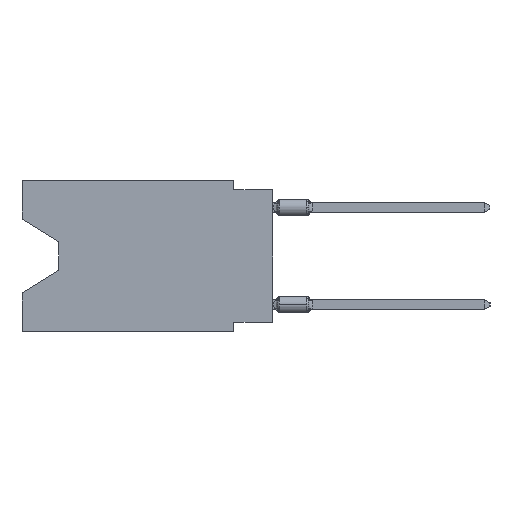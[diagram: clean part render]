
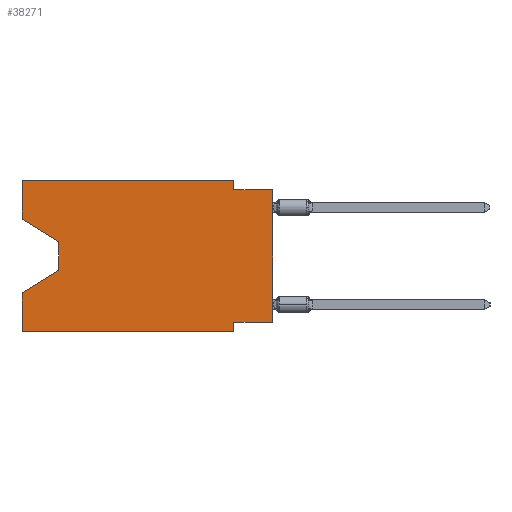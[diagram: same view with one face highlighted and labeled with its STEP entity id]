
A CAD part, left-side view. The second image highlights one B-rep face of the part: STEP entity #38271.
In plain terms, the highlighted planar face has unit normal (-1, 0, 0).
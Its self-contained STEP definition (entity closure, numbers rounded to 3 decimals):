
#84 = AXIS2_PLACEMENT_3D ( 'NONE', #37325, #18719, #42147 ) ;
#248 = EDGE_CURVE ( 'NONE', #34217, #11226, #20038, .T. ) ;
#250 = LINE ( 'NONE', #18867, #55713 ) ;
#2290 = VECTOR ( 'NONE', #35414, 1000. ) ;
#2906 = EDGE_CURVE ( 'NONE', #6430, #59969, #56478, .T. ) ;
#4871 = ORIENTED_EDGE ( 'NONE', *, *, #248, .T. ) ;
#5699 = CARTESIAN_POINT ( 'NONE',  ( 0., 0., 0. ) ) ;
#5927 = CARTESIAN_POINT ( 'NONE',  ( 0., 13.97, -4.013 ) ) ;
#6006 = LINE ( 'NONE', #5699, #39794 ) ;
#6430 = VERTEX_POINT ( 'NONE', #25200 ) ;
#6886 = EDGE_CURVE ( 'NONE', #49086, #6430, #51984, .T. ) ;
#7546 = EDGE_CURVE ( 'NONE', #26648, #34217, #13705, .T. ) ;
#8816 = DIRECTION ( 'NONE',  ( 0., 0.855, -0.519 ) ) ;
#9504 = VERTEX_POINT ( 'NONE', #32286 ) ;
#11226 = VERTEX_POINT ( 'NONE', #53431 ) ;
#12006 = DIRECTION ( 'NONE',  ( 0., 0., -1. ) ) ;
#13421 = CARTESIAN_POINT ( 'NONE',  ( 0., 2.54, -9.271 ) ) ;
#13705 = LINE ( 'NONE', #24275, #27779 ) ;
#13907 = FACE_OUTER_BOUND ( 'NONE', #61934, .T. ) ;
#14045 = CARTESIAN_POINT ( 'NONE',  ( 0., 16.383, -9.906 ) ) ;
#15239 = VECTOR ( 'NONE', #28794, 1000. ) ;
#15322 = DIRECTION ( 'NONE',  ( 0., 0., -1. ) ) ;
#15374 = VECTOR ( 'NONE', #35483, 1000. ) ;
#16225 = CARTESIAN_POINT ( 'NONE',  ( 0., 16.383, -2.546 ) ) ;
#17787 = ORIENTED_EDGE ( 'NONE', *, *, #36346, .T. ) ;
#17876 = ORIENTED_EDGE ( 'NONE', *, *, #55189, .F. ) ;
#18494 = ORIENTED_EDGE ( 'NONE', *, *, #45465, .T. ) ;
#18719 = DIRECTION ( 'NONE',  ( 1., 0., 0. ) ) ;
#18867 = CARTESIAN_POINT ( 'NONE',  ( 0., 2.54, -9.906 ) ) ;
#19535 = VERTEX_POINT ( 'NONE', #13421 ) ;
#20038 = LINE ( 'NONE', #63069, #56953 ) ;
#20681 = CARTESIAN_POINT ( 'NONE',  ( 0., 16.383, -9.906 ) ) ;
#22104 = EDGE_CURVE ( 'NONE', #9504, #36078, #6006, .T. ) ;
#22663 = ORIENTED_EDGE ( 'NONE', *, *, #22104, .T. ) ;
#22854 = CARTESIAN_POINT ( 'NONE',  ( 0., 2.54, -9.906 ) ) ;
#24275 = CARTESIAN_POINT ( 'NONE',  ( 0., 13.97, -4.013 ) ) ;
#24982 = VECTOR ( 'NONE', #48238, 1000. ) ;
#25200 = CARTESIAN_POINT ( 'NONE',  ( 0., 16.383, 0. ) ) ;
#26648 = VERTEX_POINT ( 'NONE', #5927 ) ;
#27779 = VECTOR ( 'NONE', #32630, 1000. ) ;
#28009 = EDGE_CURVE ( 'NONE', #19535, #44977, #250, .T. ) ;
#28794 = DIRECTION ( 'NONE',  ( 0., -1., 0. ) ) ;
#28834 = ORIENTED_EDGE ( 'NONE', *, *, #48474, .F. ) ;
#29597 = CARTESIAN_POINT ( 'NONE',  ( 0., 0., -0.635 ) ) ;
#30302 = CARTESIAN_POINT ( 'NONE',  ( 0., 16.383, 0. ) ) ;
#30647 = LINE ( 'NONE', #60180, #42364 ) ;
#32067 = DIRECTION ( 'NONE',  ( 0., -1., 0. ) ) ;
#32108 = LINE ( 'NONE', #30302, #2290 ) ;
#32286 = CARTESIAN_POINT ( 'NONE',  ( 0., 0., -9.271 ) ) ;
#32630 = DIRECTION ( 'NONE',  ( 0., 0., -1. ) ) ;
#33446 = CARTESIAN_POINT ( 'NONE',  ( 0., 13.97, -5.893 ) ) ;
#33474 = PLANE ( 'NONE',  #84 ) ;
#33512 = CARTESIAN_POINT ( 'NONE',  ( 0., 2.54, 0. ) ) ;
#34217 = VERTEX_POINT ( 'NONE', #33446 ) ;
#35414 = DIRECTION ( 'NONE',  ( 0., 0., 1. ) ) ;
#35483 = DIRECTION ( 'NONE',  ( 0., -0.855, -0.519 ) ) ;
#35676 = VECTOR ( 'NONE', #32067, 1000. ) ;
#36078 = VERTEX_POINT ( 'NONE', #54875 ) ;
#36346 = EDGE_CURVE ( 'NONE', #36873, #44977, #58024, .T. ) ;
#36873 = VERTEX_POINT ( 'NONE', #20681 ) ;
#37325 = CARTESIAN_POINT ( 'NONE',  ( 0., 16.383, 0. ) ) ;
#38271 = ADVANCED_FACE ( 'NONE', ( #13907 ), #33474, .F. ) ;
#39794 = VECTOR ( 'NONE', #44228, 1000. ) ;
#41596 = VECTOR ( 'NONE', #60967, 1000. ) ;
#42023 = DIRECTION ( 'NONE',  ( 0., 0., 1. ) ) ;
#42147 = DIRECTION ( 'NONE',  ( 0., 0., -1. ) ) ;
#42364 = VECTOR ( 'NONE', #12006, 1000. ) ;
#43428 = LINE ( 'NONE', #29597, #24982 ) ;
#44228 = DIRECTION ( 'NONE',  ( 0., 0., 1. ) ) ;
#44977 = VERTEX_POINT ( 'NONE', #22854 ) ;
#45465 = EDGE_CURVE ( 'NONE', #49086, #26648, #55715, .T. ) ;
#46901 = ORIENTED_EDGE ( 'NONE', *, *, #50040, .F. ) ;
#48196 = ORIENTED_EDGE ( 'NONE', *, *, #7546, .T. ) ;
#48238 = DIRECTION ( 'NONE',  ( 0., -1., 0. ) ) ;
#48474 = EDGE_CURVE ( 'NONE', #36873, #11226, #32108, .T. ) ;
#49086 = VERTEX_POINT ( 'NONE', #61565 ) ;
#50040 = EDGE_CURVE ( 'NONE', #50579, #36078, #43428, .T. ) ;
#50389 = LINE ( 'NONE', #50703, #41596 ) ;
#50579 = VERTEX_POINT ( 'NONE', #56041 ) ;
#50703 = CARTESIAN_POINT ( 'NONE',  ( 0., 0., -9.271 ) ) ;
#50971 = ORIENTED_EDGE ( 'NONE', *, *, #28009, .F. ) ;
#51021 = CARTESIAN_POINT ( 'NONE',  ( 0., 16.383, 0. ) ) ;
#51354 = VECTOR ( 'NONE', #42023, 1000. ) ;
#51984 = LINE ( 'NONE', #60986, #51354 ) ;
#53431 = CARTESIAN_POINT ( 'NONE',  ( 0., 16.383, -7.36 ) ) ;
#54875 = CARTESIAN_POINT ( 'NONE',  ( 0., 0., -0.635 ) ) ;
#55189 = EDGE_CURVE ( 'NONE', #59969, #50579, #30647, .T. ) ;
#55713 = VECTOR ( 'NONE', #15322, 1000. ) ;
#55715 = LINE ( 'NONE', #16225, #15374 ) ;
#56041 = CARTESIAN_POINT ( 'NONE',  ( 0., 2.54, -0.635 ) ) ;
#56478 = LINE ( 'NONE', #51021, #35676 ) ;
#56862 = ORIENTED_EDGE ( 'NONE', *, *, #57862, .F. ) ;
#56953 = VECTOR ( 'NONE', #8816, 1000. ) ;
#57862 = EDGE_CURVE ( 'NONE', #9504, #19535, #50389, .T. ) ;
#58017 = ORIENTED_EDGE ( 'NONE', *, *, #2906, .F. ) ;
#58024 = LINE ( 'NONE', #14045, #15239 ) ;
#58812 = ORIENTED_EDGE ( 'NONE', *, *, #6886, .F. ) ;
#59969 = VERTEX_POINT ( 'NONE', #33512 ) ;
#60180 = CARTESIAN_POINT ( 'NONE',  ( 0., 2.54, 0. ) ) ;
#60967 = DIRECTION ( 'NONE',  ( 0., 1., 0. ) ) ;
#60986 = CARTESIAN_POINT ( 'NONE',  ( 0., 16.383, 0. ) ) ;
#61565 = CARTESIAN_POINT ( 'NONE',  ( 0., 16.383, -2.546 ) ) ;
#61934 = EDGE_LOOP ( 'NONE', ( #18494, #48196, #4871, #28834, #17787, #50971, #56862, #22663, #46901, #17876, #58017, #58812 ) ) ;
#63069 = CARTESIAN_POINT ( 'NONE',  ( 0., 13.97, -5.893 ) ) ;
